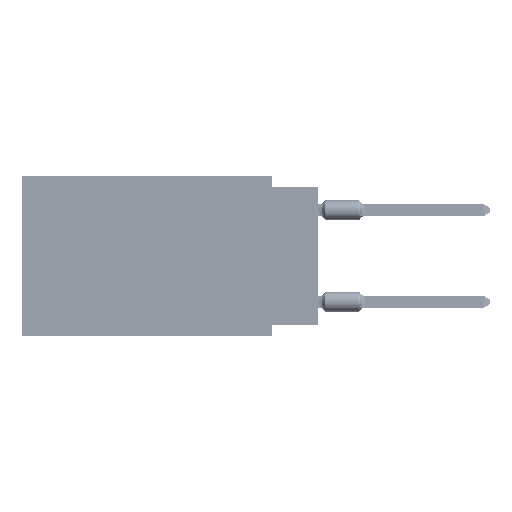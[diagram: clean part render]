
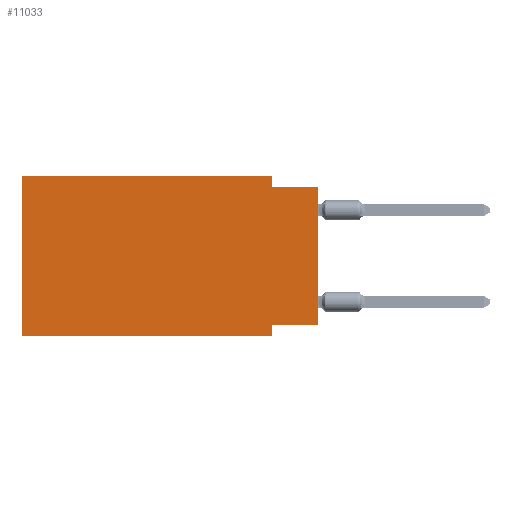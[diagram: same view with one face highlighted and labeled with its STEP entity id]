
A CAD part, left-side view. The second image highlights one B-rep face of the part: STEP entity #11033.
In plain terms, the highlighted planar face has unit normal (-1, 0, 0).
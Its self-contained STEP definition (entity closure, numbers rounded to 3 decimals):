
#659 = DIRECTION ( 'NONE',  ( 0., -1., 0. ) ) ;
#948 = DIRECTION ( 'NONE',  ( 0., 0., -1. ) ) ;
#2160 = CARTESIAN_POINT ( 'NONE',  ( 0., 2.54, -0.635 ) ) ;
#2541 = ORIENTED_EDGE ( 'NONE', *, *, #42672, .F. ) ;
#2998 = CARTESIAN_POINT ( 'NONE',  ( 0., 2.54, -8.89 ) ) ;
#7347 = LINE ( 'NONE', #93810, #37220 ) ;
#7835 = CARTESIAN_POINT ( 'NONE',  ( 0., 16.383, 0. ) ) ;
#11033 = ADVANCED_FACE ( 'NONE', ( #53101 ), #74487, .F. ) ;
#11550 = VECTOR ( 'NONE', #57769, 1000. ) ;
#12625 = EDGE_CURVE ( 'NONE', #33520, #39969, #51619, .T. ) ;
#16060 = DIRECTION ( 'NONE',  ( 1., 0., 0. ) ) ;
#19672 = VERTEX_POINT ( 'NONE', #2160 ) ;
#21781 = CARTESIAN_POINT ( 'NONE',  ( 0., 16.383, 0. ) ) ;
#23293 = EDGE_CURVE ( 'NONE', #31151, #71976, #26329, .T. ) ;
#24174 = VECTOR ( 'NONE', #79126, 1000. ) ;
#24552 = VERTEX_POINT ( 'NONE', #77211 ) ;
#24595 = EDGE_CURVE ( 'NONE', #19672, #56114, #7347, .T. ) ;
#25870 = DIRECTION ( 'NONE',  ( 0., 1., 0. ) ) ;
#26329 = LINE ( 'NONE', #47256, #41559 ) ;
#28525 = CARTESIAN_POINT ( 'NONE',  ( 0., 2.54, 0. ) ) ;
#30357 = ORIENTED_EDGE ( 'NONE', *, *, #89836, .F. ) ;
#30699 = CARTESIAN_POINT ( 'NONE',  ( 0., 0., -0.635 ) ) ;
#31151 = VERTEX_POINT ( 'NONE', #80211 ) ;
#31507 = DIRECTION ( 'NONE',  ( 0., 0., -1. ) ) ;
#33337 = EDGE_CURVE ( 'NONE', #31151, #56114, #51489, .T. ) ;
#33520 = VERTEX_POINT ( 'NONE', #21781 ) ;
#33726 = ORIENTED_EDGE ( 'NONE', *, *, #53613, .F. ) ;
#35483 = CARTESIAN_POINT ( 'NONE',  ( 0., 16.383, 0. ) ) ;
#35647 = LINE ( 'NONE', #28525, #85913 ) ;
#36822 = LINE ( 'NONE', #88117, #11550 ) ;
#37220 = VECTOR ( 'NONE', #659, 1000. ) ;
#37512 = CARTESIAN_POINT ( 'NONE',  ( 0., 2.54, 0. ) ) ;
#39969 = VERTEX_POINT ( 'NONE', #37512 ) ;
#40394 = VECTOR ( 'NONE', #52407, 1000. ) ;
#41559 = VECTOR ( 'NONE', #25870, 1000. ) ;
#42672 = EDGE_CURVE ( 'NONE', #49658, #33520, #65796, .T. ) ;
#46437 = VECTOR ( 'NONE', #31507, 1000. ) ;
#46476 = ORIENTED_EDGE ( 'NONE', *, *, #23293, .F. ) ;
#47256 = CARTESIAN_POINT ( 'NONE',  ( 0., 0., -8.255 ) ) ;
#49658 = VERTEX_POINT ( 'NONE', #58334 ) ;
#51231 = EDGE_LOOP ( 'NONE', ( #76298, #85481, #30357, #87944, #2541, #71857, #33726, #46476 ) ) ;
#51489 = LINE ( 'NONE', #87585, #40394 ) ;
#51619 = LINE ( 'NONE', #35483, #79496 ) ;
#52407 = DIRECTION ( 'NONE',  ( 0., 0., 1. ) ) ;
#53101 = FACE_OUTER_BOUND ( 'NONE', #51231, .T. ) ;
#53556 = CARTESIAN_POINT ( 'NONE',  ( 0., 16.383, 0. ) ) ;
#53613 = EDGE_CURVE ( 'NONE', #71976, #24552, #81877, .T. ) ;
#56114 = VERTEX_POINT ( 'NONE', #30699 ) ;
#57769 = DIRECTION ( 'NONE',  ( 0., -1., 0. ) ) ;
#58334 = CARTESIAN_POINT ( 'NONE',  ( 0., 16.383, -8.89 ) ) ;
#65796 = LINE ( 'NONE', #7835, #24174 ) ;
#69849 = EDGE_CURVE ( 'NONE', #49658, #24552, #36822, .T. ) ;
#71857 = ORIENTED_EDGE ( 'NONE', *, *, #69849, .T. ) ;
#71976 = VERTEX_POINT ( 'NONE', #72733 ) ;
#72733 = CARTESIAN_POINT ( 'NONE',  ( 0., 2.54, -8.255 ) ) ;
#73253 = AXIS2_PLACEMENT_3D ( 'NONE', #53556, #16060, #82085 ) ;
#74487 = PLANE ( 'NONE',  #73253 ) ;
#76298 = ORIENTED_EDGE ( 'NONE', *, *, #33337, .T. ) ;
#77211 = CARTESIAN_POINT ( 'NONE',  ( 0., 2.54, -8.89 ) ) ;
#79126 = DIRECTION ( 'NONE',  ( 0., 0., 1. ) ) ;
#79496 = VECTOR ( 'NONE', #87727, 1000. ) ;
#80211 = CARTESIAN_POINT ( 'NONE',  ( 0., 0., -8.255 ) ) ;
#81877 = LINE ( 'NONE', #2998, #46437 ) ;
#82085 = DIRECTION ( 'NONE',  ( 0., 0., -1. ) ) ;
#85481 = ORIENTED_EDGE ( 'NONE', *, *, #24595, .F. ) ;
#85913 = VECTOR ( 'NONE', #948, 1000. ) ;
#87585 = CARTESIAN_POINT ( 'NONE',  ( 0., 0., 0. ) ) ;
#87727 = DIRECTION ( 'NONE',  ( 0., -1., 0. ) ) ;
#87944 = ORIENTED_EDGE ( 'NONE', *, *, #12625, .F. ) ;
#88117 = CARTESIAN_POINT ( 'NONE',  ( 0., 16.383, -8.89 ) ) ;
#89836 = EDGE_CURVE ( 'NONE', #39969, #19672, #35647, .T. ) ;
#93810 = CARTESIAN_POINT ( 'NONE',  ( 0., 0., -0.635 ) ) ;
